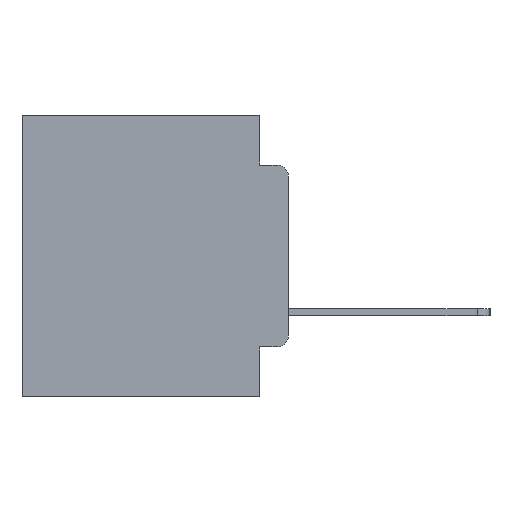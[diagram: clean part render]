
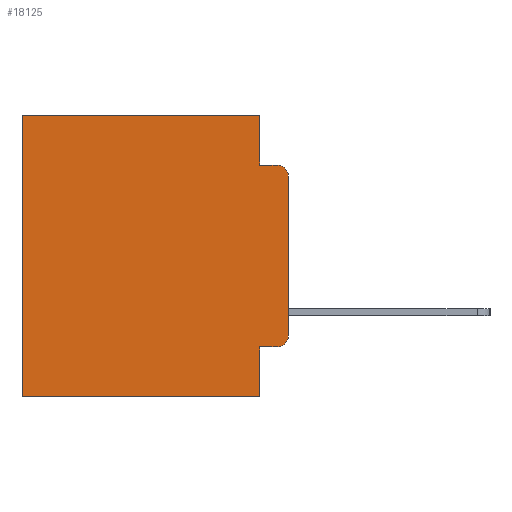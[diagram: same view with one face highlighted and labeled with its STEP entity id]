
A CAD part, left-side view. The second image highlights one B-rep face of the part: STEP entity #18125.
In plain terms, the highlighted planar face has unit normal (-1, 0, 0).
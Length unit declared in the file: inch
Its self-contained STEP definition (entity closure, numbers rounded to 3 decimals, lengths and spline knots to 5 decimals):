
#26 = EDGE_CURVE ( 'NONE', #11524, #2956, #1973, .T. ) ;
#197 = CARTESIAN_POINT ( 'NONE',  ( 0.298, 0.02, -0.3915 ) ) ;
#255 = VECTOR ( 'NONE', #9184, 39.37008 ) ;
#303 = VERTEX_POINT ( 'NONE', #11986 ) ;
#865 = CARTESIAN_POINT ( 'NONE',  ( 0.298, 0.02, -0.0885 ) ) ;
#1240 = CARTESIAN_POINT ( 'NONE',  ( 0.298, 0., -0.5 ) ) ;
#1722 = DIRECTION ( 'NONE',  ( 0., -1., 0. ) ) ;
#1895 = ORIENTED_EDGE ( 'NONE', *, *, #4954, .F. ) ;
#1973 = LINE ( 'NONE', #3473, #23074 ) ;
#2412 = CARTESIAN_POINT ( 'NONE',  ( 0.298, 0.051, -0.4115 ) ) ;
#2541 = CARTESIAN_POINT ( 'NONE',  ( 0.298, 0., 0. ) ) ;
#2609 = DIRECTION ( 'NONE',  ( 0., 0., -1. ) ) ;
#2712 = EDGE_CURVE ( 'NONE', #22909, #13141, #15105, .T. ) ;
#2956 = VERTEX_POINT ( 'NONE', #6091 ) ;
#3121 = CARTESIAN_POINT ( 'NONE',  ( 0.298, 0.473, -0.5 ) ) ;
#3473 = CARTESIAN_POINT ( 'NONE',  ( 0.298, 0., 0. ) ) ;
#3914 = LINE ( 'NONE', #4090, #9554 ) ;
#4090 = CARTESIAN_POINT ( 'NONE',  ( 0.298, 0.051, 0. ) ) ;
#4197 = VERTEX_POINT ( 'NONE', #19091 ) ;
#4226 = FACE_OUTER_BOUND ( 'NONE', #27430, .T. ) ;
#4696 = EDGE_CURVE ( 'NONE', #4197, #25248, #23911, .T. ) ;
#4780 = DIRECTION ( 'NONE',  ( 0., 0., -1. ) ) ;
#4898 = EDGE_CURVE ( 'NONE', #4197, #25642, #18596, .T. ) ;
#4929 = AXIS2_PLACEMENT_3D ( 'NONE', #8683, #23614, #10835 ) ;
#4943 = EDGE_CURVE ( 'NONE', #303, #25642, #27100, .T. ) ;
#4954 = EDGE_CURVE ( 'NONE', #11524, #303, #3914, .T. ) ;
#5040 = EDGE_CURVE ( 'NONE', #2956, #13141, #12245, .T. ) ;
#5045 = EDGE_CURVE ( 'NONE', #25784, #22909, #5687, .T. ) ;
#5047 = EDGE_CURVE ( 'NONE', #25784, #19817, #11582, .T. ) ;
#5050 = ORIENTED_EDGE ( 'NONE', *, *, #4898, .T. ) ;
#5075 = EDGE_CURVE ( 'NONE', #19817, #25248, #21597, .T. ) ;
#5687 = LINE ( 'NONE', #24076, #27764 ) ;
#5912 = CARTESIAN_POINT ( 'NONE',  ( 0.298, 0.051, -0.4115 ) ) ;
#6091 = CARTESIAN_POINT ( 'NONE',  ( 0.298, 0.473, 0. ) ) ;
#6303 = CARTESIAN_POINT ( 'NONE',  ( 0.298, 0.051, -0.0885 ) ) ;
#6673 = CARTESIAN_POINT ( 'NONE',  ( 0.298, 0.051, -0.5 ) ) ;
#7839 = CARTESIAN_POINT ( 'NONE',  ( 0.298, 0.051, 0. ) ) ;
#8011 = CARTESIAN_POINT ( 'NONE',  ( 0.298, 0.02, -0.1085 ) ) ;
#8681 = VECTOR ( 'NONE', #15804, 39.37008 ) ;
#8683 = CARTESIAN_POINT ( 'NONE',  ( 0.298, 0., 0. ) ) ;
#8929 = ORIENTED_EDGE ( 'NONE', *, *, #5045, .F. ) ;
#9184 = DIRECTION ( 'NONE',  ( 0., -1., 0. ) ) ;
#9554 = VECTOR ( 'NONE', #21477, 39.37008 ) ;
#10188 = DIRECTION ( 'NONE',  ( 0., 0., -1. ) ) ;
#10835 = DIRECTION ( 'NONE',  ( 0., 0., -1. ) ) ;
#11387 = ORIENTED_EDGE ( 'NONE', *, *, #5075, .T. ) ;
#11524 = VERTEX_POINT ( 'NONE', #7839 ) ;
#11582 = LINE ( 'NONE', #2412, #255 ) ;
#11986 = CARTESIAN_POINT ( 'NONE',  ( 0.298, 0.051, -0.0885 ) ) ;
#12245 = LINE ( 'NONE', #28088, #23601 ) ;
#12336 = ORIENTED_EDGE ( 'NONE', *, *, #4943, .F. ) ;
#12675 = AXIS2_PLACEMENT_3D ( 'NONE', #8011, #22962, #10188 ) ;
#13141 = VERTEX_POINT ( 'NONE', #3121 ) ;
#13414 = DIRECTION ( 'NONE',  ( 0., 0., -1. ) ) ;
#15105 = LINE ( 'NONE', #1240, #8681 ) ;
#15172 = CARTESIAN_POINT ( 'NONE',  ( 0.298, 0., -0.3915 ) ) ;
#15197 = CARTESIAN_POINT ( 'NONE',  ( 0.298, 0.02, -0.4115 ) ) ;
#15299 = VECTOR ( 'NONE', #1722, 39.37008 ) ;
#15697 = DIRECTION ( 'NONE',  ( 0., 0., -1. ) ) ;
#15804 = DIRECTION ( 'NONE',  ( 0., 1., 0. ) ) ;
#15882 = DIRECTION ( 'NONE',  ( -1., 0., 0. ) ) ;
#17234 = PLANE ( 'NONE',  #4929 ) ;
#18125 = ADVANCED_FACE ( 'NONE', ( #4226 ), #17234, .F. ) ;
#18596 = CIRCLE ( 'NONE', #12675, 0.02 ) ;
#19091 = CARTESIAN_POINT ( 'NONE',  ( 0.298, 0., -0.1085 ) ) ;
#19817 = VERTEX_POINT ( 'NONE', #15197 ) ;
#20026 = ORIENTED_EDGE ( 'NONE', *, *, #26, .T. ) ;
#20050 = ORIENTED_EDGE ( 'NONE', *, *, #5047, .T. ) ;
#20364 = ORIENTED_EDGE ( 'NONE', *, *, #4696, .F. ) ;
#20536 = DIRECTION ( 'NONE',  ( 0., 1., 0. ) ) ;
#21477 = DIRECTION ( 'NONE',  ( 0., 0., -1. ) ) ;
#21597 = CIRCLE ( 'NONE', #23559, 0.02 ) ;
#22016 = ORIENTED_EDGE ( 'NONE', *, *, #2712, .F. ) ;
#22909 = VERTEX_POINT ( 'NONE', #6673 ) ;
#22962 = DIRECTION ( 'NONE',  ( -1., 0., 0. ) ) ;
#23074 = VECTOR ( 'NONE', #20536, 39.37008 ) ;
#23559 = AXIS2_PLACEMENT_3D ( 'NONE', #197, #15882, #2609 ) ;
#23601 = VECTOR ( 'NONE', #13414, 39.37008 ) ;
#23614 = DIRECTION ( 'NONE',  ( 1., 0., 0. ) ) ;
#23911 = LINE ( 'NONE', #2541, #28048 ) ;
#24076 = CARTESIAN_POINT ( 'NONE',  ( 0.298, 0.051, 0. ) ) ;
#25248 = VERTEX_POINT ( 'NONE', #15172 ) ;
#25642 = VERTEX_POINT ( 'NONE', #865 ) ;
#25784 = VERTEX_POINT ( 'NONE', #5912 ) ;
#26920 = ORIENTED_EDGE ( 'NONE', *, *, #5040, .T. ) ;
#27100 = LINE ( 'NONE', #6303, #15299 ) ;
#27430 = EDGE_LOOP ( 'NONE', ( #20364, #5050, #12336, #1895, #20026, #26920, #22016, #8929, #20050, #11387 ) ) ;
#27764 = VECTOR ( 'NONE', #15697, 39.37008 ) ;
#28048 = VECTOR ( 'NONE', #4780, 39.37008 ) ;
#28088 = CARTESIAN_POINT ( 'NONE',  ( 0.298, 0.473, 0. ) ) ;
